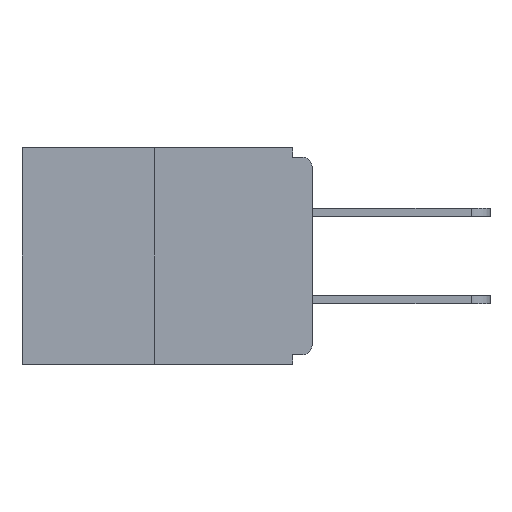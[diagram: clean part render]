
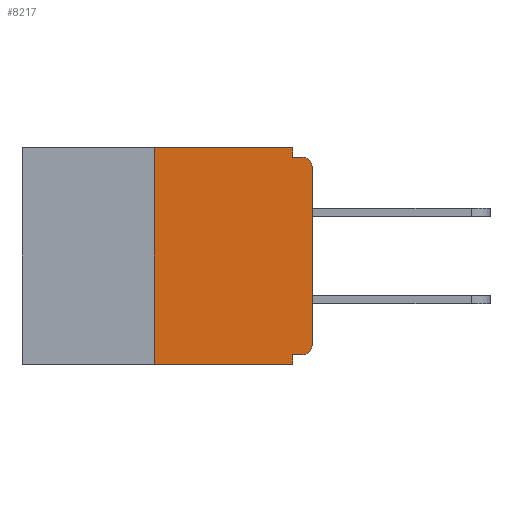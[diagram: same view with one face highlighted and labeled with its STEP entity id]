
A CAD part, left-side view. The second image highlights one B-rep face of the part: STEP entity #8217.
In plain terms, the highlighted planar face has unit normal (-1, 0, 0).
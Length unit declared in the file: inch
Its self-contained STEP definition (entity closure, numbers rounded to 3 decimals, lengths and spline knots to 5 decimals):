
#893 = DIRECTION ( 'NONE',  ( 0., 0., -1. ) ) ;
#1123 = DIRECTION ( 'NONE',  ( 0., -1., 0. ) ) ;
#1127 = ORIENTED_EDGE ( 'NONE', *, *, #13344, .F. ) ;
#1345 = DIRECTION ( 'NONE',  ( -1., 0., 0. ) ) ;
#1459 = ORIENTED_EDGE ( 'NONE', *, *, #18205, .T. ) ;
#1809 = DIRECTION ( 'NONE',  ( 0., 0., 1. ) ) ;
#1916 = ORIENTED_EDGE ( 'NONE', *, *, #4244, .F. ) ;
#2656 = VERTEX_POINT ( 'NONE', #4671 ) ;
#3013 = DIRECTION ( 'NONE',  ( 1., 0., 0. ) ) ;
#3887 = LINE ( 'NONE', #8632, #11822 ) ;
#3985 = VERTEX_POINT ( 'NONE', #26301 ) ;
#4043 = VERTEX_POINT ( 'NONE', #22065 ) ;
#4124 = ORIENTED_EDGE ( 'NONE', *, *, #11177, .T. ) ;
#4244 = EDGE_CURVE ( 'NONE', #9924, #25604, #11160, .T. ) ;
#4290 = AXIS2_PLACEMENT_3D ( 'NONE', #24927, #3013, #893 ) ;
#4671 = CARTESIAN_POINT ( 'NONE',  ( 0., 0., -0.03 ) ) ;
#4758 = CARTESIAN_POINT ( 'NONE',  ( 0., 0.25, 0. ) ) ;
#5312 = VERTEX_POINT ( 'NONE', #5686 ) ;
#5686 = CARTESIAN_POINT ( 'NONE',  ( 0., 0.031, -0.343 ) ) ;
#6006 = CIRCLE ( 'NONE', #24209, 0.015 ) ;
#6187 = VECTOR ( 'NONE', #6441, 39.37008 ) ;
#6219 = FACE_OUTER_BOUND ( 'NONE', #23193, .T. ) ;
#6441 = DIRECTION ( 'NONE',  ( 0., 0., -1. ) ) ;
#6883 = LINE ( 'NONE', #9036, #29538 ) ;
#7961 = ORIENTED_EDGE ( 'NONE', *, *, #8642, .F. ) ;
#8096 = VERTEX_POINT ( 'NONE', #22623 ) ;
#8217 = ADVANCED_FACE ( 'NONE', ( #6219 ), #17933, .F. ) ;
#8482 = LINE ( 'NONE', #16039, #6187 ) ;
#8500 = EDGE_CURVE ( 'NONE', #25604, #8096, #8482, .T. ) ;
#8632 = CARTESIAN_POINT ( 'NONE',  ( 0., 0., 0. ) ) ;
#8642 = EDGE_CURVE ( 'NONE', #3985, #26945, #10327, .T. ) ;
#8873 = DIRECTION ( 'NONE',  ( 0., -1., 0. ) ) ;
#9036 = CARTESIAN_POINT ( 'NONE',  ( 0., 0.031, -0.343 ) ) ;
#9152 = CARTESIAN_POINT ( 'NONE',  ( 0., 0.015, -0.015 ) ) ;
#9924 = VERTEX_POINT ( 'NONE', #4758 ) ;
#10225 = ORIENTED_EDGE ( 'NONE', *, *, #15166, .T. ) ;
#10327 = LINE ( 'NONE', #21857, #16397 ) ;
#10649 = DIRECTION ( 'NONE',  ( -1., 0., 0. ) ) ;
#11160 = LINE ( 'NONE', #30270, #27356 ) ;
#11177 = EDGE_CURVE ( 'NONE', #2656, #19142, #16989, .T. ) ;
#11822 = VECTOR ( 'NONE', #13165, 39.37008 ) ;
#12602 = VERTEX_POINT ( 'NONE', #30960 ) ;
#13165 = DIRECTION ( 'NONE',  ( 0., 0., 1. ) ) ;
#13344 = EDGE_CURVE ( 'NONE', #8096, #19142, #15710, .T. ) ;
#13796 = ORIENTED_EDGE ( 'NONE', *, *, #8500, .F. ) ;
#14668 = EDGE_CURVE ( 'NONE', #12602, #5312, #26955, .T. ) ;
#14689 = LINE ( 'NONE', #18835, #20015 ) ;
#15166 = EDGE_CURVE ( 'NONE', #4043, #2656, #3887, .T. ) ;
#15710 = LINE ( 'NONE', #22700, #24034 ) ;
#15830 = CARTESIAN_POINT ( 'NONE',  ( 0., 0.46, -0.343 ) ) ;
#15909 = CARTESIAN_POINT ( 'NONE',  ( 0., 0.031, 0. ) ) ;
#16039 = CARTESIAN_POINT ( 'NONE',  ( 0., 0.031, 0. ) ) ;
#16397 = VECTOR ( 'NONE', #24190, 39.37008 ) ;
#16989 = CIRCLE ( 'NONE', #25244, 0.015 ) ;
#17933 = PLANE ( 'NONE',  #4290 ) ;
#18205 = EDGE_CURVE ( 'NONE', #3985, #4043, #6006, .T. ) ;
#18280 = DIRECTION ( 'NONE',  ( 0., 0., -1. ) ) ;
#18835 = CARTESIAN_POINT ( 'NONE',  ( 0., 0.25, 0. ) ) ;
#19142 = VERTEX_POINT ( 'NONE', #9152 ) ;
#19443 = VECTOR ( 'NONE', #8873, 39.37008 ) ;
#20015 = VECTOR ( 'NONE', #1809, 39.37008 ) ;
#21023 = CARTESIAN_POINT ( 'NONE',  ( 0., 0.015, -0.03 ) ) ;
#21857 = CARTESIAN_POINT ( 'NONE',  ( 0., 0., -0.328 ) ) ;
#22065 = CARTESIAN_POINT ( 'NONE',  ( 0., 0., -0.313 ) ) ;
#22623 = CARTESIAN_POINT ( 'NONE',  ( 0., 0.031, -0.015 ) ) ;
#22700 = CARTESIAN_POINT ( 'NONE',  ( 0., 0., -0.015 ) ) ;
#22818 = CARTESIAN_POINT ( 'NONE',  ( 0., 0.015, -0.313 ) ) ;
#23193 = EDGE_LOOP ( 'NONE', ( #1916, #26469, #27179, #28167, #7961, #1459, #10225, #4124, #1127, #13796 ) ) ;
#23916 = EDGE_CURVE ( 'NONE', #26945, #5312, #6883, .T. ) ;
#24034 = VECTOR ( 'NONE', #1123, 39.37008 ) ;
#24190 = DIRECTION ( 'NONE',  ( 0., 1., 0. ) ) ;
#24209 = AXIS2_PLACEMENT_3D ( 'NONE', #22818, #10649, #29866 ) ;
#24927 = CARTESIAN_POINT ( 'NONE',  ( 0., 0.46, 0. ) ) ;
#25244 = AXIS2_PLACEMENT_3D ( 'NONE', #21023, #1345, #18280 ) ;
#25604 = VERTEX_POINT ( 'NONE', #15909 ) ;
#25922 = DIRECTION ( 'NONE',  ( 0., 0., -1. ) ) ;
#26109 = EDGE_CURVE ( 'NONE', #12602, #9924, #14689, .T. ) ;
#26301 = CARTESIAN_POINT ( 'NONE',  ( 0., 0.015, -0.328 ) ) ;
#26469 = ORIENTED_EDGE ( 'NONE', *, *, #26109, .F. ) ;
#26945 = VERTEX_POINT ( 'NONE', #29085 ) ;
#26955 = LINE ( 'NONE', #15830, #19443 ) ;
#27179 = ORIENTED_EDGE ( 'NONE', *, *, #14668, .T. ) ;
#27356 = VECTOR ( 'NONE', #28043, 39.37008 ) ;
#28043 = DIRECTION ( 'NONE',  ( 0., -1., 0. ) ) ;
#28167 = ORIENTED_EDGE ( 'NONE', *, *, #23916, .F. ) ;
#29085 = CARTESIAN_POINT ( 'NONE',  ( 0., 0.031, -0.328 ) ) ;
#29538 = VECTOR ( 'NONE', #25922, 39.37008 ) ;
#29866 = DIRECTION ( 'NONE',  ( 0., 0., -1. ) ) ;
#30270 = CARTESIAN_POINT ( 'NONE',  ( 0., 0.46, 0. ) ) ;
#30960 = CARTESIAN_POINT ( 'NONE',  ( 0., 0.25, -0.343 ) ) ;
